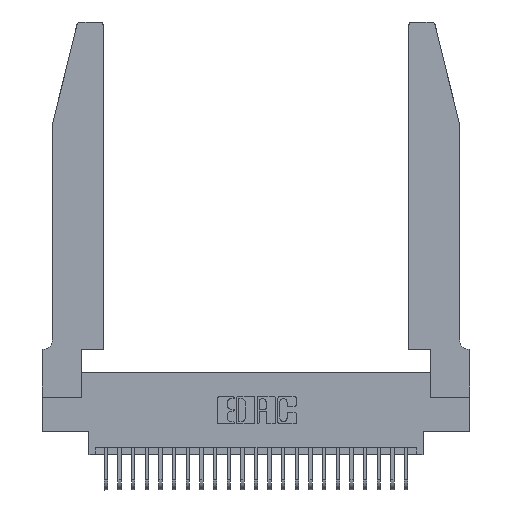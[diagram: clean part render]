
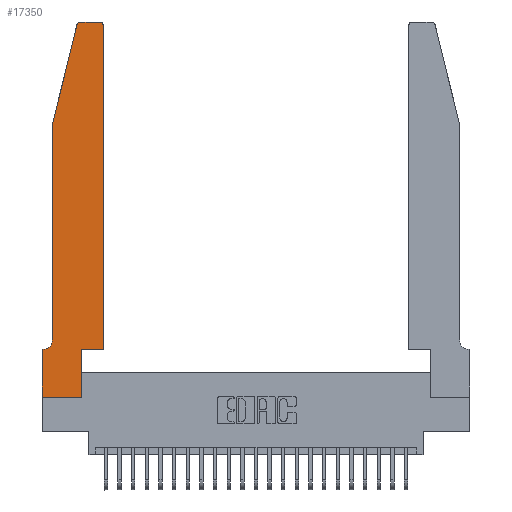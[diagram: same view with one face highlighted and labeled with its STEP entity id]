
A CAD part, top view. The second image highlights one B-rep face of the part: STEP entity #17350.
In plain terms, the highlighted planar face has unit normal (0, 0, 1).
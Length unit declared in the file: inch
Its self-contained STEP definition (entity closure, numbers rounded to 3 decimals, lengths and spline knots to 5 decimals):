
#56 = AXIS2_PLACEMENT_3D ( 'NONE', #21168, #9772, #23059 ) ;
#127 = CARTESIAN_POINT ( 'NONE',  ( 0.0055, 0.35, 0.37 ) ) ;
#128 = DIRECTION ( 'NONE',  ( 0., 1., 0. ) ) ;
#623 = LINE ( 'NONE', #13693, #1303 ) ;
#659 = CARTESIAN_POINT ( 'NONE',  ( 0., 0.35, 0.37 ) ) ;
#745 = VERTEX_POINT ( 'NONE', #22333 ) ;
#874 = EDGE_CURVE ( 'NONE', #22884, #22768, #14497, .T. ) ;
#942 = VERTEX_POINT ( 'NONE', #2116 ) ;
#1113 = CARTESIAN_POINT ( 'NONE',  ( 0.2865, 0.35, 0.37 ) ) ;
#1303 = VECTOR ( 'NONE', #128, 39.37008 ) ;
#1391 = VERTEX_POINT ( 'NONE', #5886 ) ;
#1472 = CARTESIAN_POINT ( 'NONE',  ( 0.0755, 0.42, 0.37 ) ) ;
#1506 = VECTOR ( 'NONE', #2046, 39.37008 ) ;
#1844 = VERTEX_POINT ( 'NONE', #1472 ) ;
#2046 = DIRECTION ( 'NONE',  ( 1., 0., 0. ) ) ;
#2116 = CARTESIAN_POINT ( 'NONE',  ( 0.25487, 2.72718, 0.37 ) ) ;
#2122 = VECTOR ( 'NONE', #9873, 39.37008 ) ;
#2735 = DIRECTION ( 'NONE',  ( 0., 0., 1. ) ) ;
#2847 = ORIENTED_EDGE ( 'NONE', *, *, #11739, .T. ) ;
#3336 = DIRECTION ( 'NONE',  ( -1., 0., 0. ) ) ;
#3856 = VECTOR ( 'NONE', #3336, 39.37008 ) ;
#3880 = VECTOR ( 'NONE', #15717, 39.37008 ) ;
#3908 = ORIENTED_EDGE ( 'NONE', *, *, #17635, .T. ) ;
#3945 = VERTEX_POINT ( 'NONE', #5036 ) ;
#4163 = CARTESIAN_POINT ( 'NONE',  ( 0., 0., 0.37 ) ) ;
#4563 = DIRECTION ( 'NONE',  ( -1., 0., 0. ) ) ;
#4883 = ORIENTED_EDGE ( 'NONE', *, *, #6175, .T. ) ;
#5036 = CARTESIAN_POINT ( 'NONE',  ( 0.2865, 0.35, 0.37 ) ) ;
#5270 = AXIS2_PLACEMENT_3D ( 'NONE', #18132, #6611, #20022 ) ;
#5472 = ORIENTED_EDGE ( 'NONE', *, *, #13622, .T. ) ;
#5886 = CARTESIAN_POINT ( 'NONE',  ( 0.284, 2.75, 0.37 ) ) ;
#6175 = EDGE_CURVE ( 'NONE', #745, #3945, #23473, .T. ) ;
#6611 = DIRECTION ( 'NONE',  ( 0., 0., -1. ) ) ;
#6853 = EDGE_CURVE ( 'NONE', #8689, #745, #9139, .T. ) ;
#7233 = EDGE_CURVE ( 'NONE', #18211, #22884, #623, .T. ) ;
#7517 = CARTESIAN_POINT ( 'NONE',  ( 0.0755, 2., 0.37 ) ) ;
#7545 = DIRECTION ( 'NONE',  ( 1., 0., 0. ) ) ;
#8004 = CIRCLE ( 'NONE', #16794, 0.03 ) ;
#8388 = AXIS2_PLACEMENT_3D ( 'NONE', #17139, #19038, #7545 ) ;
#8689 = VERTEX_POINT ( 'NONE', #20169 ) ;
#8743 = VECTOR ( 'NONE', #11444, 39.37008 ) ;
#8856 = ORIENTED_EDGE ( 'NONE', *, *, #11697, .T. ) ;
#9044 = LINE ( 'NONE', #4163, #3880 ) ;
#9139 = LINE ( 'NONE', #22137, #18723 ) ;
#9758 = EDGE_CURVE ( 'NONE', #1391, #942, #8004, .T. ) ;
#9772 = DIRECTION ( 'NONE',  ( 0., 0., 1. ) ) ;
#9873 = DIRECTION ( 'NONE',  ( -0.239, -0.971, 0. ) ) ;
#10649 = LINE ( 'NONE', #13743, #2122 ) ;
#11444 = DIRECTION ( 'NONE',  ( 0., -1., 0. ) ) ;
#11697 = EDGE_CURVE ( 'NONE', #3945, #18211, #16306, .T. ) ;
#11739 = EDGE_CURVE ( 'NONE', #942, #12617, #10649, .T. ) ;
#12242 = ORIENTED_EDGE ( 'NONE', *, *, #13355, .T. ) ;
#12617 = VERTEX_POINT ( 'NONE', #18607 ) ;
#12699 = ORIENTED_EDGE ( 'NONE', *, *, #17612, .T. ) ;
#12903 = CARTESIAN_POINT ( 'NONE',  ( 0.4205, 2.75, 0.37 ) ) ;
#12914 = VERTEX_POINT ( 'NONE', #127 ) ;
#13001 = CARTESIAN_POINT ( 'NONE',  ( 0.2605, 2.75, 0.37 ) ) ;
#13318 = PLANE ( 'NONE',  #8388 ) ;
#13355 = EDGE_CURVE ( 'NONE', #22768, #1391, #24196, .T. ) ;
#13622 = EDGE_CURVE ( 'NONE', #14334, #8689, #9044, .T. ) ;
#13665 = CARTESIAN_POINT ( 'NONE',  ( 0.4505, 0.35, 0.37 ) ) ;
#13693 = CARTESIAN_POINT ( 'NONE',  ( 0.4505, 0.35, 0.37 ) ) ;
#13743 = CARTESIAN_POINT ( 'NONE',  ( 0.0755, 2., 0.37 ) ) ;
#14017 = VECTOR ( 'NONE', #14641, 39.37008 ) ;
#14149 = ORIENTED_EDGE ( 'NONE', *, *, #9758, .T. ) ;
#14330 = CARTESIAN_POINT ( 'NONE',  ( 0.284, 2.72, 0.37 ) ) ;
#14334 = VERTEX_POINT ( 'NONE', #659 ) ;
#14472 = LINE ( 'NONE', #16132, #18913 ) ;
#14497 = CIRCLE ( 'NONE', #56, 0.03 ) ;
#14641 = DIRECTION ( 'NONE',  ( 0., 1., 0. ) ) ;
#15137 = EDGE_LOOP ( 'NONE', ( #12242, #14149, #2847, #21813, #3908, #12699, #5472, #22557, #4883, #8856, #23601, #22911 ) ) ;
#15717 = DIRECTION ( 'NONE',  ( 0., -1., 0. ) ) ;
#16132 = CARTESIAN_POINT ( 'NONE',  ( 0.0755, 0.35, 0.37 ) ) ;
#16233 = DIRECTION ( 'NONE',  ( 1., 0., 0. ) ) ;
#16306 = LINE ( 'NONE', #13665, #1506 ) ;
#16794 = AXIS2_PLACEMENT_3D ( 'NONE', #14330, #2735, #16233 ) ;
#17047 = CARTESIAN_POINT ( 'NONE',  ( 0.4505, 2.72, 0.37 ) ) ;
#17139 = CARTESIAN_POINT ( 'NONE',  ( 0., 0.35, 0.37 ) ) ;
#17350 = ADVANCED_FACE ( 'NONE', ( #24831 ), #13318, .T. ) ;
#17612 = EDGE_CURVE ( 'NONE', #12914, #14334, #14472, .T. ) ;
#17635 = EDGE_CURVE ( 'NONE', #1844, #12914, #23936, .T. ) ;
#18132 = CARTESIAN_POINT ( 'NONE',  ( 0.0055, 0.42, 0.37 ) ) ;
#18211 = VERTEX_POINT ( 'NONE', #23449 ) ;
#18607 = CARTESIAN_POINT ( 'NONE',  ( 0.0755, 2., 0.37 ) ) ;
#18723 = VECTOR ( 'NONE', #24029, 39.37008 ) ;
#18913 = VECTOR ( 'NONE', #4563, 39.37008 ) ;
#19038 = DIRECTION ( 'NONE',  ( 0., 0., 1. ) ) ;
#20022 = DIRECTION ( 'NONE',  ( -1., 0., 0. ) ) ;
#20169 = CARTESIAN_POINT ( 'NONE',  ( 0., 0., 0.37 ) ) ;
#21168 = CARTESIAN_POINT ( 'NONE',  ( 0.4205, 2.72, 0.37 ) ) ;
#21813 = ORIENTED_EDGE ( 'NONE', *, *, #23544, .T. ) ;
#22137 = CARTESIAN_POINT ( 'NONE',  ( 0., 0., 0.37 ) ) ;
#22333 = CARTESIAN_POINT ( 'NONE',  ( 0.2865, 0., 0.37 ) ) ;
#22557 = ORIENTED_EDGE ( 'NONE', *, *, #6853, .T. ) ;
#22768 = VERTEX_POINT ( 'NONE', #12903 ) ;
#22884 = VERTEX_POINT ( 'NONE', #17047 ) ;
#22911 = ORIENTED_EDGE ( 'NONE', *, *, #874, .T. ) ;
#23059 = DIRECTION ( 'NONE',  ( 1., 0., 0. ) ) ;
#23346 = LINE ( 'NONE', #7517, #8743 ) ;
#23449 = CARTESIAN_POINT ( 'NONE',  ( 0.4505, 0.35, 0.37 ) ) ;
#23473 = LINE ( 'NONE', #1113, #14017 ) ;
#23544 = EDGE_CURVE ( 'NONE', #12617, #1844, #23346, .T. ) ;
#23601 = ORIENTED_EDGE ( 'NONE', *, *, #7233, .T. ) ;
#23936 = CIRCLE ( 'NONE', #5270, 0.07 ) ;
#24029 = DIRECTION ( 'NONE',  ( 1., 0., 0. ) ) ;
#24196 = LINE ( 'NONE', #13001, #3856 ) ;
#24831 = FACE_OUTER_BOUND ( 'NONE', #15137, .T. ) ;
